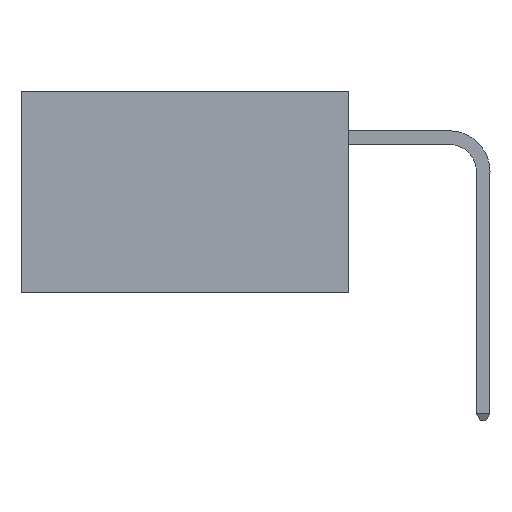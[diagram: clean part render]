
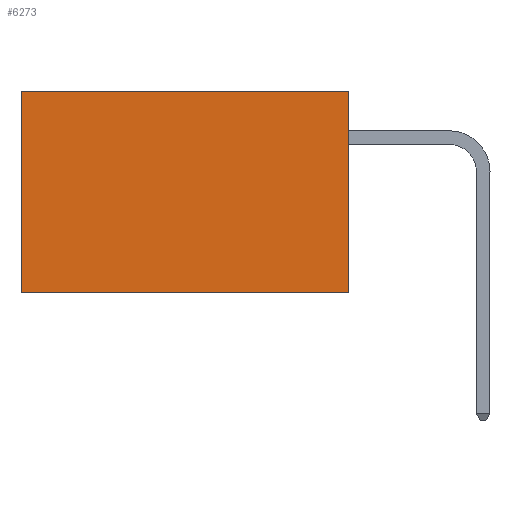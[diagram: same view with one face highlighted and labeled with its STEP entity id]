
A CAD part, left-side view. The second image highlights one B-rep face of the part: STEP entity #6273.
In plain terms, the highlighted planar face has unit normal (-1, 0, 0).
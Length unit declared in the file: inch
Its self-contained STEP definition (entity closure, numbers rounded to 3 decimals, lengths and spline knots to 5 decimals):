
#556 = LINE ( 'NONE', #4010, #5919 ) ;
#597 = EDGE_CURVE ( 'NONE', #9990, #10667, #2736, .T. ) ;
#1801 = CARTESIAN_POINT ( 'NONE',  ( 0.2875, 0., 0. ) ) ;
#2736 = LINE ( 'NONE', #8973, #7453 ) ;
#3026 = VECTOR ( 'NONE', #3680, 39.37008 ) ;
#3680 = DIRECTION ( 'NONE',  ( 0., 0., -1. ) ) ;
#4010 = CARTESIAN_POINT ( 'NONE',  ( 0.2875, 0.6, 0. ) ) ;
#4233 = FACE_OUTER_BOUND ( 'NONE', #8990, .T. ) ;
#5579 = LINE ( 'NONE', #12055, #7395 ) ;
#5919 = VECTOR ( 'NONE', #9591, 39.37008 ) ;
#6014 = EDGE_CURVE ( 'NONE', #11708, #9777, #5579, .T. ) ;
#6273 = ADVANCED_FACE ( 'NONE', ( #4233 ), #10911, .F. ) ;
#6412 = DIRECTION ( 'NONE',  ( 0., 0., -1. ) ) ;
#6685 = DIRECTION ( 'NONE',  ( 0., 1., 0. ) ) ;
#6907 = CARTESIAN_POINT ( 'NONE',  ( 0.2875, 0.6, -0.37 ) ) ;
#7395 = VECTOR ( 'NONE', #11022, 39.37008 ) ;
#7453 = VECTOR ( 'NONE', #6685, 39.37008 ) ;
#8371 = EDGE_CURVE ( 'NONE', #9777, #10667, #556, .T. ) ;
#8941 = CARTESIAN_POINT ( 'NONE',  ( 0.2875, 0., 0. ) ) ;
#8973 = CARTESIAN_POINT ( 'NONE',  ( 0.2875, 0., -0.37 ) ) ;
#8990 = EDGE_LOOP ( 'NONE', ( #10077, #12047, #10340, #10621 ) ) ;
#9012 = AXIS2_PLACEMENT_3D ( 'NONE', #8941, #12243, #6412 ) ;
#9255 = CARTESIAN_POINT ( 'NONE',  ( 0.2875, 0., 0. ) ) ;
#9591 = DIRECTION ( 'NONE',  ( 0., 0., -1. ) ) ;
#9777 = VERTEX_POINT ( 'NONE', #11821 ) ;
#9990 = VERTEX_POINT ( 'NONE', #11283 ) ;
#10077 = ORIENTED_EDGE ( 'NONE', *, *, #8371, .T. ) ;
#10177 = LINE ( 'NONE', #9255, #3026 ) ;
#10340 = ORIENTED_EDGE ( 'NONE', *, *, #10373, .F. ) ;
#10373 = EDGE_CURVE ( 'NONE', #11708, #9990, #10177, .T. ) ;
#10621 = ORIENTED_EDGE ( 'NONE', *, *, #6014, .T. ) ;
#10667 = VERTEX_POINT ( 'NONE', #6907 ) ;
#10911 = PLANE ( 'NONE',  #9012 ) ;
#11022 = DIRECTION ( 'NONE',  ( 0., 1., 0. ) ) ;
#11283 = CARTESIAN_POINT ( 'NONE',  ( 0.2875, 0., -0.37 ) ) ;
#11708 = VERTEX_POINT ( 'NONE', #1801 ) ;
#11821 = CARTESIAN_POINT ( 'NONE',  ( 0.2875, 0.6, 0. ) ) ;
#12047 = ORIENTED_EDGE ( 'NONE', *, *, #597, .F. ) ;
#12055 = CARTESIAN_POINT ( 'NONE',  ( 0.2875, 0., 0. ) ) ;
#12243 = DIRECTION ( 'NONE',  ( 1., 0., 0. ) ) ;
